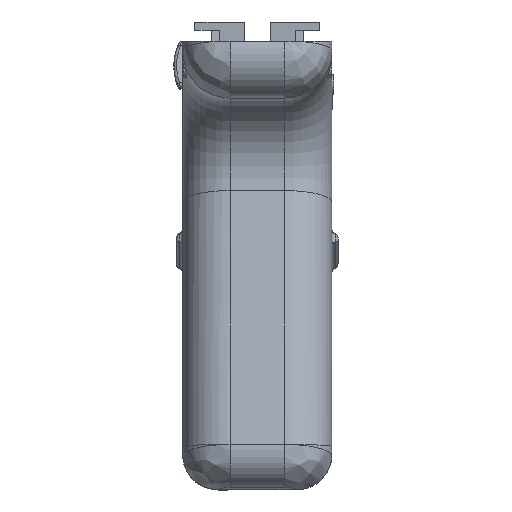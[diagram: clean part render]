
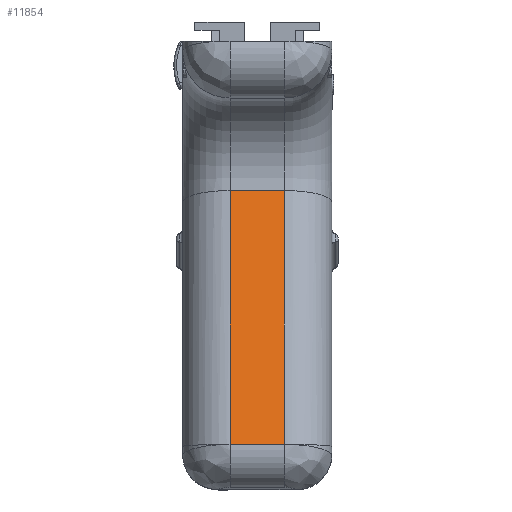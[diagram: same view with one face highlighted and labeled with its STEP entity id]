
A CAD part, front view. The second image highlights one B-rep face of the part: STEP entity #11854.
In plain terms, the highlighted face is planar.
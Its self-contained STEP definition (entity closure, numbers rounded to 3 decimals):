
#886=PLANE('',#12965);
#1483=FACE_OUTER_BOUND('',#2161,.T.);
#2161=EDGE_LOOP('',(#10655,#10656,#10657,#10658));
#3110=LINE('',#21602,#4207);
#3264=LINE('',#22447,#4361);
#3265=LINE('',#22450,#4362);
#3266=LINE('',#22451,#4363);
#4207=VECTOR('',#15558,10.);
#4361=VECTOR('',#15958,10.);
#4362=VECTOR('',#15961,10.);
#4363=VECTOR('',#15962,10.);
#5679=VERTEX_POINT('',#21598);
#5680=VERTEX_POINT('',#21600);
#5815=VERTEX_POINT('',#22425);
#5818=VERTEX_POINT('',#22449);
#7260=EDGE_CURVE('',#5679,#5680,#3110,.T.);
#7484=EDGE_CURVE('',#5679,#5815,#3264,.T.);
#7485=EDGE_CURVE('',#5818,#5680,#3265,.T.);
#7486=EDGE_CURVE('',#5815,#5818,#3266,.T.);
#10655=ORIENTED_EDGE('',*,*,#7485,.F.);
#10656=ORIENTED_EDGE('',*,*,#7486,.F.);
#10657=ORIENTED_EDGE('',*,*,#7484,.F.);
#10658=ORIENTED_EDGE('',*,*,#7260,.T.);
#11854=ADVANCED_FACE('',(#1483),#886,.T.);
#12965=AXIS2_PLACEMENT_3D('',#22448,#15959,#15960);
#15558=DIRECTION('',(0.,-0.249,0.969));
#15958=DIRECTION('',(-1.,0.,0.));
#15959=DIRECTION('center_axis',(0.,-0.969,
-0.249));
#15960=DIRECTION('ref_axis',(0.,-0.249,0.969));
#15961=DIRECTION('',(1.,0.,0.));
#15962=DIRECTION('',(0.,-0.249,0.969));
#21598=CARTESIAN_POINT('',(13.45,-71.634,19.877));
#21600=CARTESIAN_POINT('',(13.45,-83.628,66.536));
#21602=CARTESIAN_POINT('',(13.45,-83.554,66.245));
#22425=CARTESIAN_POINT('',(3.45,-71.634,19.877));
#22447=CARTESIAN_POINT('',(22.175,-71.634,19.877));
#22448=CARTESIAN_POINT('Origin',(22.175,-71.634,19.877));
#22449=CARTESIAN_POINT('',(3.45,-83.628,66.536));
#22450=CARTESIAN_POINT('',(22.175,-83.628,66.536));
#22451=CARTESIAN_POINT('',(3.45,-83.554,66.245));
